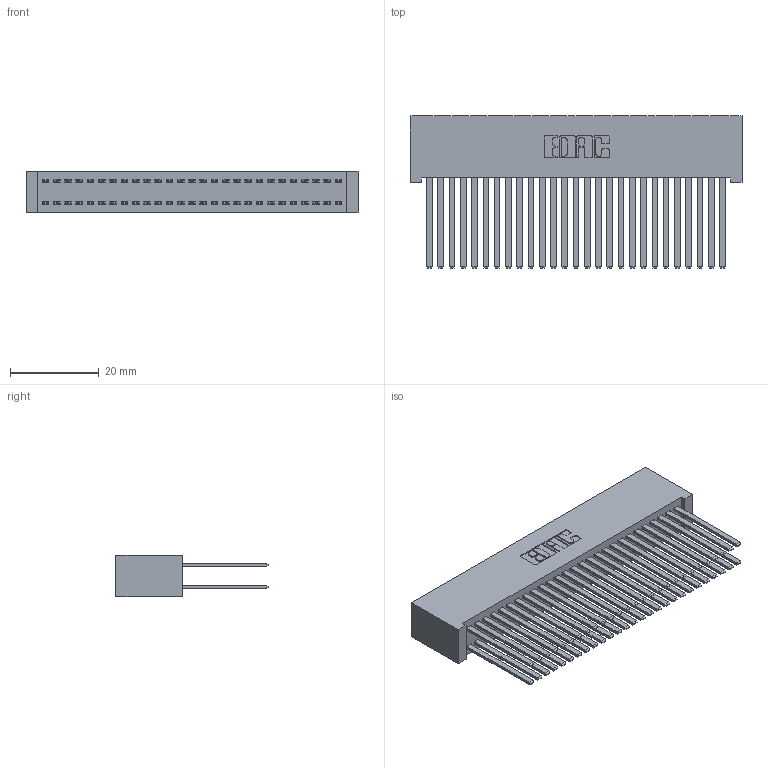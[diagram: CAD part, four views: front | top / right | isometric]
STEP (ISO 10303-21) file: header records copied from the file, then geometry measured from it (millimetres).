
FILE_DESCRIPTION (( 'STEP AP203' ), '1' );
FILE_NAME ('342-054-544-201.STEP', '2018-08-13T00:38:57', ( '' ), ( '' ), 'SwSTEP 2.0', 'SolidWorks 2016', '' );
FILE_SCHEMA (( 'CONFIG_CONTROL_DESIGN' ));
Length unit declared in the file: inch
Products named in the file (3): 342 Part_Lugless; 345-292-001_345-293-144; 342-054-544-201
Assembly tree (55 placements, depth 2):
  342-054-544-201
    342 Part_Lugless
    345-292-001_345-293-144  x54
Bounding box: 74.83 x 34.3 x 9.4 mm (x, y, z)
Volume: 7848.8 mm3; surface area: 14948.9 mm2
Topology: 55 solids, 55 shells, 2586 faces, 7673 edges, 5042 vertices
Faces by surface type: plane 1790, cylinder 796
Entity records: 18717 total; most frequent: CARTESIAN_POINT 3114, ORIENTED_EDGE 3050, DIRECTION 2677, EDGE_CURVE 1525, VECTOR 1409, LINE 1409, VERTEX_POINT 1014, AXIS2_PLACEMENT_3D 634
